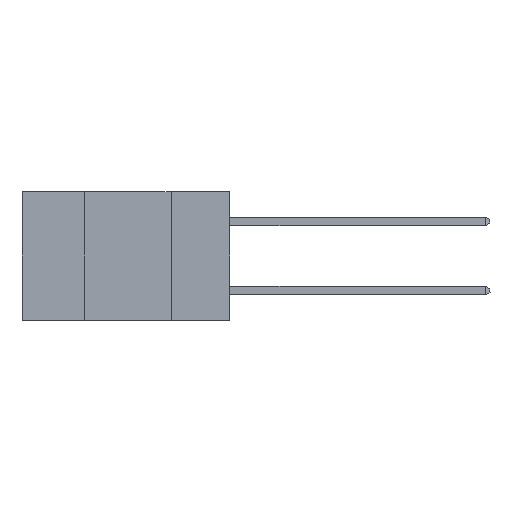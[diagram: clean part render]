
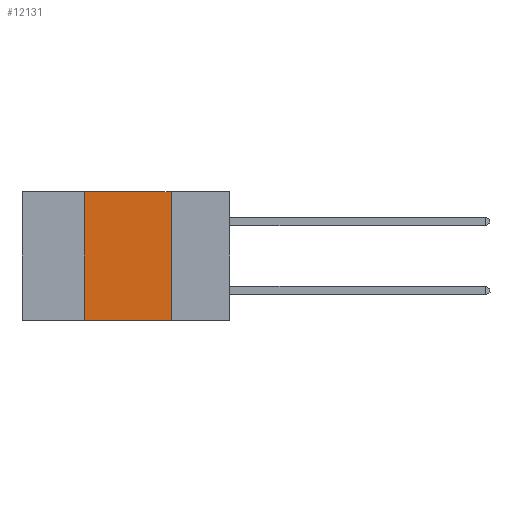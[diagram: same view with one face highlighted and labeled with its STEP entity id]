
A CAD part, left-side view. The second image highlights one B-rep face of the part: STEP entity #12131.
In plain terms, the highlighted planar face has unit normal (-1, 0, 0).
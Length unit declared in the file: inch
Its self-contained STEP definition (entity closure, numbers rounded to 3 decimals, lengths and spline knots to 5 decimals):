
#401 = DIRECTION ( 'NONE',  ( 0., 0., -1. ) ) ;
#435 = ORIENTED_EDGE ( 'NONE', *, *, #10599, .F. ) ;
#536 = EDGE_LOOP ( 'NONE', ( #435, #12240, #2561, #10716 ) ) ;
#663 = DIRECTION ( 'NONE',  ( 0., 0., 1. ) ) ;
#977 = CARTESIAN_POINT ( 'NONE',  ( 0., 0.6, -0.37 ) ) ;
#1694 = VERTEX_POINT ( 'NONE', #2989 ) ;
#1899 = LINE ( 'NONE', #9394, #8591 ) ;
#2561 = ORIENTED_EDGE ( 'NONE', *, *, #10635, .F. ) ;
#2614 = VECTOR ( 'NONE', #10638, 39.37008 ) ;
#2919 = EDGE_CURVE ( 'NONE', #4037, #5617, #9787, .T. ) ;
#2928 = VECTOR ( 'NONE', #9359, 39.37008 ) ;
#2989 = CARTESIAN_POINT ( 'NONE',  ( 0., 0.42, 0. ) ) ;
#3200 = CARTESIAN_POINT ( 'NONE',  ( 0., 0.6, 0. ) ) ;
#4037 = VERTEX_POINT ( 'NONE', #12362 ) ;
#4184 = PLANE ( 'NONE',  #10828 ) ;
#5403 = CARTESIAN_POINT ( 'NONE',  ( 0., 0.6, 0. ) ) ;
#5504 = DIRECTION ( 'NONE',  ( 0., 0., -1. ) ) ;
#5508 = VERTEX_POINT ( 'NONE', #7049 ) ;
#5617 = VERTEX_POINT ( 'NONE', #7431 ) ;
#5810 = LINE ( 'NONE', #5403, #2928 ) ;
#7049 = CARTESIAN_POINT ( 'NONE',  ( 0., 0.17, 0. ) ) ;
#7431 = CARTESIAN_POINT ( 'NONE',  ( 0., 0.17, -0.37 ) ) ;
#7878 = EDGE_CURVE ( 'NONE', #1694, #5508, #5810, .T. ) ;
#8280 = FACE_OUTER_BOUND ( 'NONE', #536, .T. ) ;
#8591 = VECTOR ( 'NONE', #5504, 39.37008 ) ;
#9359 = DIRECTION ( 'NONE',  ( 0., -1., 0. ) ) ;
#9394 = CARTESIAN_POINT ( 'NONE',  ( 0., 0.17, 0. ) ) ;
#9787 = LINE ( 'NONE', #977, #2614 ) ;
#10003 = DIRECTION ( 'NONE',  ( 1., 0., 0. ) ) ;
#10107 = LINE ( 'NONE', #12226, #10552 ) ;
#10552 = VECTOR ( 'NONE', #663, 39.37008 ) ;
#10599 = EDGE_CURVE ( 'NONE', #5508, #5617, #1899, .T. ) ;
#10635 = EDGE_CURVE ( 'NONE', #4037, #1694, #10107, .T. ) ;
#10638 = DIRECTION ( 'NONE',  ( 0., -1., 0. ) ) ;
#10716 = ORIENTED_EDGE ( 'NONE', *, *, #2919, .T. ) ;
#10828 = AXIS2_PLACEMENT_3D ( 'NONE', #3200, #10003, #401 ) ;
#12131 = ADVANCED_FACE ( 'NONE', ( #8280 ), #4184, .F. ) ;
#12226 = CARTESIAN_POINT ( 'NONE',  ( 0., 0.42, 0. ) ) ;
#12240 = ORIENTED_EDGE ( 'NONE', *, *, #7878, .F. ) ;
#12362 = CARTESIAN_POINT ( 'NONE',  ( 0., 0.42, -0.37 ) ) ;
